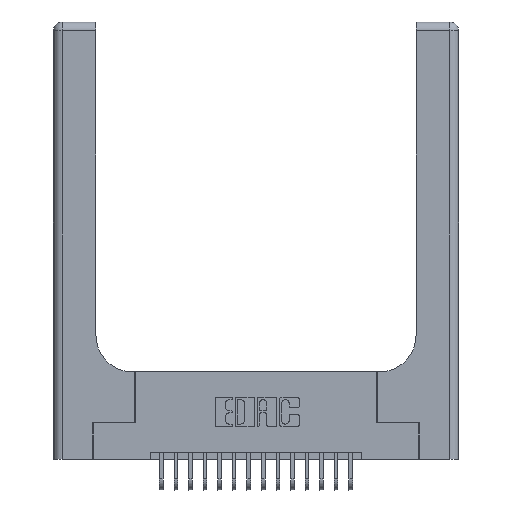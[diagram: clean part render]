
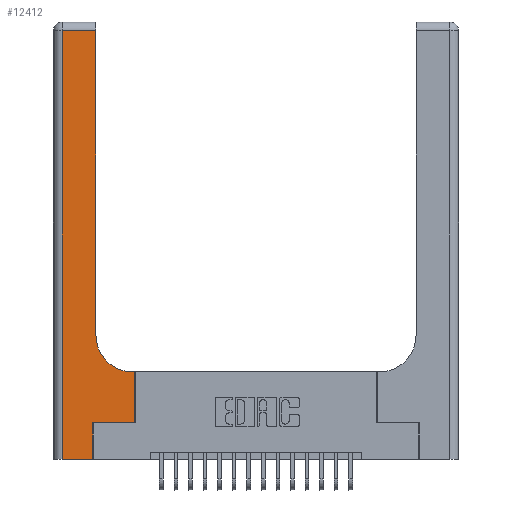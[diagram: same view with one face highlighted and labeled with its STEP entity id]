
A CAD part, top view. The second image highlights one B-rep face of the part: STEP entity #12412.
In plain terms, the highlighted planar face has unit normal (0, 0, 1).
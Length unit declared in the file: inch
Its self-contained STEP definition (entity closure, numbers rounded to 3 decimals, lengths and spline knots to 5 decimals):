
#842 = ORIENTED_EDGE ( 'NONE', *, *, #12611, .T. ) ;
#1463 = CARTESIAN_POINT ( 'NONE',  ( 0.5415, 0.85, 0.37 ) ) ;
#1533 = VECTOR ( 'NONE', #10424, 39.37008 ) ;
#1571 = CARTESIAN_POINT ( 'NONE',  ( 0.269, 0., 0.37 ) ) ;
#2192 = EDGE_CURVE ( 'NONE', #8117, #21488, #3282, .T. ) ;
#2613 = CARTESIAN_POINT ( 'NONE',  ( 0.06, 3., 0.37 ) ) ;
#2993 = EDGE_CURVE ( 'NONE', #7915, #15773, #21494, .T. ) ;
#3152 = ORIENTED_EDGE ( 'NONE', *, *, #5044, .T. ) ;
#3282 = LINE ( 'NONE', #12456, #19456 ) ;
#3542 = CARTESIAN_POINT ( 'NONE',  ( 0.2915, 0.6, 0.37 ) ) ;
#4155 = FACE_OUTER_BOUND ( 'NONE', #7011, .T. ) ;
#4430 = DIRECTION ( 'NONE',  ( -1., 0., 0. ) ) ;
#4916 = LINE ( 'NONE', #17180, #1533 ) ;
#5044 = EDGE_CURVE ( 'NONE', #7078, #9019, #16679, .T. ) ;
#5072 = CARTESIAN_POINT ( 'NONE',  ( 0.2915, 0.85, 0.37 ) ) ;
#5094 = LINE ( 'NONE', #6415, #20745 ) ;
#6084 = LINE ( 'NONE', #3542, #13344 ) ;
#6348 = VECTOR ( 'NONE', #12333, 39.37008 ) ;
#6415 = CARTESIAN_POINT ( 'NONE',  ( 0.5585, 0.25, 0.37 ) ) ;
#6699 = VECTOR ( 'NONE', #10897, 39.37008 ) ;
#7011 = EDGE_LOOP ( 'NONE', ( #21561, #15690, #20542, #842, #20987, #10395, #13543, #13931, #3152 ) ) ;
#7078 = VERTEX_POINT ( 'NONE', #16006 ) ;
#7664 = AXIS2_PLACEMENT_3D ( 'NONE', #1463, #17979, #12879 ) ;
#7915 = VERTEX_POINT ( 'NONE', #14199 ) ;
#8117 = VERTEX_POINT ( 'NONE', #1571 ) ;
#8677 = VERTEX_POINT ( 'NONE', #12044 ) ;
#9019 = VERTEX_POINT ( 'NONE', #5072 ) ;
#9075 = EDGE_CURVE ( 'NONE', #8677, #20717, #5094, .T. ) ;
#9618 = DIRECTION ( 'NONE',  ( 0., 1., 0. ) ) ;
#10395 = ORIENTED_EDGE ( 'NONE', *, *, #19706, .T. ) ;
#10424 = DIRECTION ( 'NONE',  ( 0., 1., 0. ) ) ;
#10483 = CARTESIAN_POINT ( 'NONE',  ( 0.06, 2.94, 0.37 ) ) ;
#10897 = DIRECTION ( 'NONE',  ( 1., 0., 0. ) ) ;
#10920 = VECTOR ( 'NONE', #16609, 39.37008 ) ;
#11091 = DIRECTION ( 'NONE',  ( -1., 0., 0. ) ) ;
#12044 = CARTESIAN_POINT ( 'NONE',  ( 0.5585, 0.25, 0.37 ) ) ;
#12333 = DIRECTION ( 'NONE',  ( 0., -1., 0. ) ) ;
#12412 = ADVANCED_FACE ( 'NONE', ( #4155 ), #14384, .F. ) ;
#12456 = CARTESIAN_POINT ( 'NONE',  ( 0.269, 0., 0.37 ) ) ;
#12611 = EDGE_CURVE ( 'NONE', #18834, #8117, #16110, .T. ) ;
#12797 = EDGE_CURVE ( 'NONE', #9019, #7915, #4916, .T. ) ;
#12879 = DIRECTION ( 'NONE',  ( 1., 0., 0. ) ) ;
#13344 = VECTOR ( 'NONE', #16861, 39.37008 ) ;
#13403 = CARTESIAN_POINT ( 'NONE',  ( 0., 0., 0.37 ) ) ;
#13543 = ORIENTED_EDGE ( 'NONE', *, *, #9075, .T. ) ;
#13931 = ORIENTED_EDGE ( 'NONE', *, *, #16278, .T. ) ;
#14199 = CARTESIAN_POINT ( 'NONE',  ( 0.2915, 2.94, 0.37 ) ) ;
#14384 = PLANE ( 'NONE',  #18442 ) ;
#15690 = ORIENTED_EDGE ( 'NONE', *, *, #2993, .T. ) ;
#15773 = VERTEX_POINT ( 'NONE', #10483 ) ;
#15807 = DIRECTION ( 'NONE',  ( 0., 0., -1. ) ) ;
#15901 = DIRECTION ( 'NONE',  ( 0., 1., 0. ) ) ;
#15956 = EDGE_CURVE ( 'NONE', #15773, #18834, #15973, .T. ) ;
#15973 = LINE ( 'NONE', #2613, #6348 ) ;
#16006 = CARTESIAN_POINT ( 'NONE',  ( 0.5415, 0.6, 0.37 ) ) ;
#16052 = CARTESIAN_POINT ( 'NONE',  ( 0.269, 0.25, 0.37 ) ) ;
#16110 = LINE ( 'NONE', #13403, #10920 ) ;
#16278 = EDGE_CURVE ( 'NONE', #20717, #7078, #6084, .T. ) ;
#16609 = DIRECTION ( 'NONE',  ( 1., 0., 0. ) ) ;
#16679 = CIRCLE ( 'NONE', #7664, 0.25 ) ;
#16745 = CARTESIAN_POINT ( 'NONE',  ( 0.269, 0.25, 0.37 ) ) ;
#16840 = LINE ( 'NONE', #16052, #6699 ) ;
#16861 = DIRECTION ( 'NONE',  ( -1., 0., 0. ) ) ;
#17180 = CARTESIAN_POINT ( 'NONE',  ( 0.2915, 3., 0.37 ) ) ;
#17979 = DIRECTION ( 'NONE',  ( 0., 0., -1. ) ) ;
#18012 = CARTESIAN_POINT ( 'NONE',  ( 0.5585, 0.6, 0.37 ) ) ;
#18430 = CARTESIAN_POINT ( 'NONE',  ( 0.06, 0., 0.37 ) ) ;
#18442 = AXIS2_PLACEMENT_3D ( 'NONE', #21091, #15807, #11091 ) ;
#18834 = VERTEX_POINT ( 'NONE', #18430 ) ;
#19456 = VECTOR ( 'NONE', #15901, 39.37008 ) ;
#19706 = EDGE_CURVE ( 'NONE', #21488, #8677, #16840, .T. ) ;
#20542 = ORIENTED_EDGE ( 'NONE', *, *, #15956, .T. ) ;
#20717 = VERTEX_POINT ( 'NONE', #18012 ) ;
#20725 = VECTOR ( 'NONE', #4430, 39.37008 ) ;
#20745 = VECTOR ( 'NONE', #9618, 39.37008 ) ;
#20987 = ORIENTED_EDGE ( 'NONE', *, *, #2192, .T. ) ;
#20989 = CARTESIAN_POINT ( 'NONE',  ( 0., 2.94, 0.37 ) ) ;
#21091 = CARTESIAN_POINT ( 'NONE',  ( 0., 3., 0.37 ) ) ;
#21488 = VERTEX_POINT ( 'NONE', #16745 ) ;
#21494 = LINE ( 'NONE', #20989, #20725 ) ;
#21561 = ORIENTED_EDGE ( 'NONE', *, *, #12797, .T. ) ;
